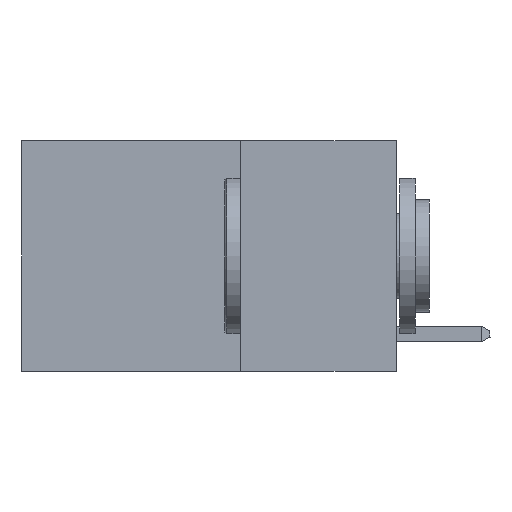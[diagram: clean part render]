
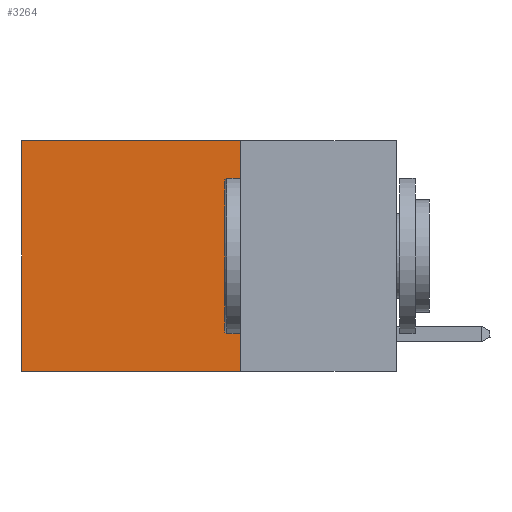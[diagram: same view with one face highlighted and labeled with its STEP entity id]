
A CAD part, left-side view. The second image highlights one B-rep face of the part: STEP entity #3264.
In plain terms, the highlighted planar face has unit normal (-1, 0, 0).
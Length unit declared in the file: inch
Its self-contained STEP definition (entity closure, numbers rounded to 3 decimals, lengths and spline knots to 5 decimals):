
#474 = DIRECTION ( 'NONE',  ( 0., 0., -1. ) ) ;
#525 = DIRECTION ( 'NONE',  ( 1., 0., 0. ) ) ;
#545 = PLANE ( 'NONE',  #14240 ) ;
#622 = CARTESIAN_POINT ( 'NONE',  ( 0.2625, 0.25, 0. ) ) ;
#1499 = VERTEX_POINT ( 'NONE', #16538 ) ;
#2404 = VECTOR ( 'NONE', #3300, 39.37008 ) ;
#2854 = VERTEX_POINT ( 'NONE', #3946 ) ;
#3264 = ADVANCED_FACE ( 'NONE', ( #4813 ), #545, .F. ) ;
#3300 = DIRECTION ( 'NONE',  ( 0., 0., -1. ) ) ;
#3946 = CARTESIAN_POINT ( 'NONE',  ( 0.2625, 0.25, -0.37 ) ) ;
#4813 = FACE_OUTER_BOUND ( 'NONE', #6624, .T. ) ;
#5616 = CARTESIAN_POINT ( 'NONE',  ( 0.2625, 0.25, 0. ) ) ;
#6624 = EDGE_LOOP ( 'NONE', ( #13960, #8793, #14895, #19322 ) ) ;
#6741 = LINE ( 'NONE', #13031, #2404 ) ;
#7274 = DIRECTION ( 'NONE',  ( 0., 0., -1. ) ) ;
#7384 = EDGE_CURVE ( 'NONE', #2854, #13852, #12248, .T. ) ;
#7388 = EDGE_CURVE ( 'NONE', #17765, #2854, #7461, .T. ) ;
#7461 = LINE ( 'NONE', #5616, #15532 ) ;
#8793 = ORIENTED_EDGE ( 'NONE', *, *, #7384, .F. ) ;
#10424 = CARTESIAN_POINT ( 'NONE',  ( 0.2625, 0.25, -0.37 ) ) ;
#11364 = LINE ( 'NONE', #20527, #15151 ) ;
#12248 = LINE ( 'NONE', #10424, #20264 ) ;
#12550 = DIRECTION ( 'NONE',  ( 0., 1., 0. ) ) ;
#12652 = EDGE_CURVE ( 'NONE', #1499, #13852, #6741, .T. ) ;
#13031 = CARTESIAN_POINT ( 'NONE',  ( 0.2625, 0.6, 0. ) ) ;
#13345 = CARTESIAN_POINT ( 'NONE',  ( 0.2625, 0.25, 0. ) ) ;
#13852 = VERTEX_POINT ( 'NONE', #14445 ) ;
#13960 = ORIENTED_EDGE ( 'NONE', *, *, #12652, .T. ) ;
#14240 = AXIS2_PLACEMENT_3D ( 'NONE', #622, #525, #474 ) ;
#14445 = CARTESIAN_POINT ( 'NONE',  ( 0.2625, 0.6, -0.37 ) ) ;
#14895 = ORIENTED_EDGE ( 'NONE', *, *, #7388, .F. ) ;
#15151 = VECTOR ( 'NONE', #12550, 39.37008 ) ;
#15532 = VECTOR ( 'NONE', #7274, 39.37008 ) ;
#16538 = CARTESIAN_POINT ( 'NONE',  ( 0.2625, 0.6, 0. ) ) ;
#17765 = VERTEX_POINT ( 'NONE', #13345 ) ;
#18980 = EDGE_CURVE ( 'NONE', #17765, #1499, #11364, .T. ) ;
#19322 = ORIENTED_EDGE ( 'NONE', *, *, #18980, .T. ) ;
#20051 = DIRECTION ( 'NONE',  ( 0., 1., 0. ) ) ;
#20264 = VECTOR ( 'NONE', #20051, 39.37008 ) ;
#20527 = CARTESIAN_POINT ( 'NONE',  ( 0.2625, 0.25, 0. ) ) ;
